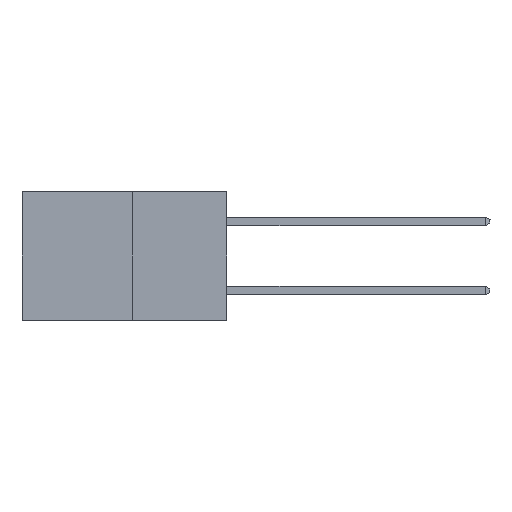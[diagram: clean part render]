
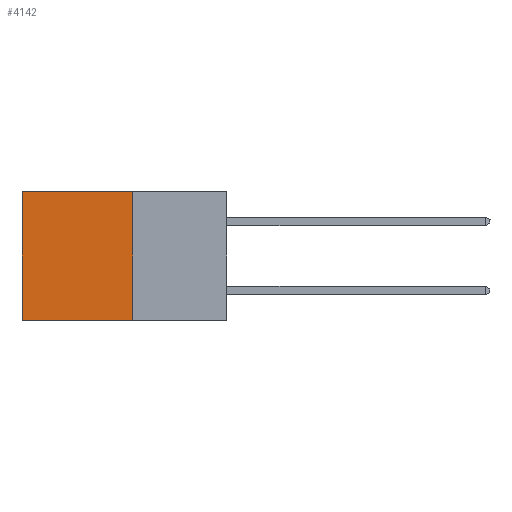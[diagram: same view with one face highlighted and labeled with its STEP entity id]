
A CAD part, left-side view. The second image highlights one B-rep face of the part: STEP entity #4142.
In plain terms, the highlighted planar face has unit normal (-1, 0, 0).
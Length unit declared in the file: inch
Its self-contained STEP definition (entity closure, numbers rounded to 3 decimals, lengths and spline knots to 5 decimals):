
#385 = CARTESIAN_POINT ( 'NONE',  ( 0.277, 0.27, 0. ) ) ;
#619 = CARTESIAN_POINT ( 'NONE',  ( 0.277, 0.59, -0.37 ) ) ;
#799 = LINE ( 'NONE', #5164, #6337 ) ;
#1049 = VECTOR ( 'NONE', #5740, 39.37008 ) ;
#1108 = VECTOR ( 'NONE', #12335, 39.37008 ) ;
#2012 = CARTESIAN_POINT ( 'NONE',  ( 0.277, 0.27, -0.37 ) ) ;
#2565 = EDGE_CURVE ( 'NONE', #8713, #10471, #799, .T. ) ;
#2587 = CARTESIAN_POINT ( 'NONE',  ( 0.277, 0.27, -0.37 ) ) ;
#2619 = DIRECTION ( 'NONE',  ( 0., 0., -1. ) ) ;
#2655 = ORIENTED_EDGE ( 'NONE', *, *, #4737, .F. ) ;
#3017 = VERTEX_POINT ( 'NONE', #6296 ) ;
#3968 = EDGE_CURVE ( 'NONE', #4795, #8713, #4303, .T. ) ;
#4142 = ADVANCED_FACE ( 'NONE', ( #12770 ), #9203, .F. ) ;
#4303 = LINE ( 'NONE', #4756, #1108 ) ;
#4530 = DIRECTION ( 'NONE',  ( 0., 0., -1. ) ) ;
#4564 = DIRECTION ( 'NONE',  ( 1., 0., 0. ) ) ;
#4737 = EDGE_CURVE ( 'NONE', #4795, #3017, #7306, .T. ) ;
#4756 = CARTESIAN_POINT ( 'NONE',  ( 0.277, 0.27, 0. ) ) ;
#4795 = VERTEX_POINT ( 'NONE', #385 ) ;
#5164 = CARTESIAN_POINT ( 'NONE',  ( 0.277, 0.59, -0.37 ) ) ;
#5223 = ORIENTED_EDGE ( 'NONE', *, *, #2565, .T. ) ;
#5740 = DIRECTION ( 'NONE',  ( 0., 1., 0. ) ) ;
#5761 = CARTESIAN_POINT ( 'NONE',  ( 0.277, 0.27, -0.37 ) ) ;
#6296 = CARTESIAN_POINT ( 'NONE',  ( 0.277, 0.27, -0.37 ) ) ;
#6337 = VECTOR ( 'NONE', #4530, 39.37008 ) ;
#7285 = LINE ( 'NONE', #5761, #1049 ) ;
#7306 = LINE ( 'NONE', #2012, #13235 ) ;
#7429 = CARTESIAN_POINT ( 'NONE',  ( 0.277, 0.59, 0. ) ) ;
#8181 = ORIENTED_EDGE ( 'NONE', *, *, #8958, .F. ) ;
#8713 = VERTEX_POINT ( 'NONE', #7429 ) ;
#8958 = EDGE_CURVE ( 'NONE', #3017, #10471, #7285, .T. ) ;
#9203 = PLANE ( 'NONE',  #13230 ) ;
#10471 = VERTEX_POINT ( 'NONE', #619 ) ;
#11681 = ORIENTED_EDGE ( 'NONE', *, *, #3968, .T. ) ;
#12335 = DIRECTION ( 'NONE',  ( 0., 1., 0. ) ) ;
#12770 = FACE_OUTER_BOUND ( 'NONE', #13493, .T. ) ;
#13230 = AXIS2_PLACEMENT_3D ( 'NONE', #2587, #4564, #13398 ) ;
#13235 = VECTOR ( 'NONE', #2619, 39.37008 ) ;
#13398 = DIRECTION ( 'NONE',  ( 0., 0., -1. ) ) ;
#13493 = EDGE_LOOP ( 'NONE', ( #5223, #8181, #2655, #11681 ) ) ;
